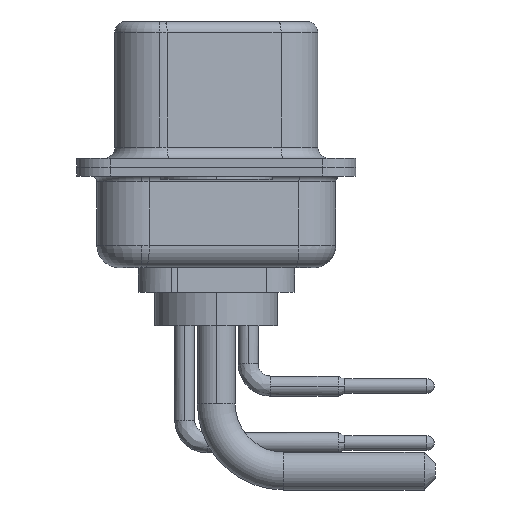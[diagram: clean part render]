
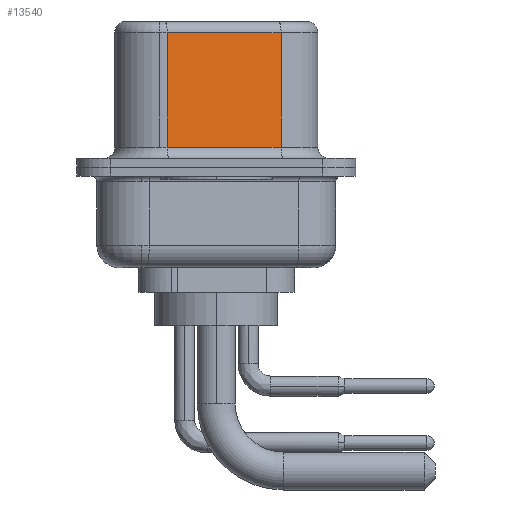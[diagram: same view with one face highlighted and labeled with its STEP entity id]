
A CAD part, left-side view. The second image highlights one B-rep face of the part: STEP entity #13540.
In plain terms, the highlighted planar face has unit normal (-0.985, -0.174, 0).
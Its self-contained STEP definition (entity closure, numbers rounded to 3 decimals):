
#1412 = EDGE_CURVE ( 'NONE', #9887, #16896, #6601, .T. ) ;
#1560 = DIRECTION ( 'NONE',  ( 0., 0., -1. ) ) ;
#3458 = PLANE ( 'NONE',  #9472 ) ;
#3875 = DIRECTION ( 'NONE',  ( -0.174, 0.985, 0. ) ) ;
#4397 = DIRECTION ( 'NONE',  ( 0.174, -0.985, 0. ) ) ;
#4495 = CARTESIAN_POINT ( 'NONE',  ( 3.68, 2.203, 6.02 ) ) ;
#4924 = CARTESIAN_POINT ( 'NONE',  ( 4.58, -2.897, 6.52 ) ) ;
#5695 = ORIENTED_EDGE ( 'NONE', *, *, #16134, .T. ) ;
#6601 = LINE ( 'NONE', #11292, #7530 ) ;
#6937 = ORIENTED_EDGE ( 'NONE', *, *, #1412, .T. ) ;
#7530 = VECTOR ( 'NONE', #15975, 1000. ) ;
#7934 = CARTESIAN_POINT ( 'NONE',  ( 4.58, -2.897, 6.02 ) ) ;
#8263 = DIRECTION ( 'NONE',  ( 0.985, 0.174, 0. ) ) ;
#9199 = ORIENTED_EDGE ( 'NONE', *, *, #12507, .T. ) ;
#9436 = VECTOR ( 'NONE', #4397, 1000. ) ;
#9472 = AXIS2_PLACEMENT_3D ( 'NONE', #16198, #8263, #3875 ) ;
#9713 = LINE ( 'NONE', #4924, #14267 ) ;
#9887 = VERTEX_POINT ( 'NONE', #7934 ) ;
#10927 = VERTEX_POINT ( 'NONE', #16264 ) ;
#11241 = ORIENTED_EDGE ( 'NONE', *, *, #18923, .F. ) ;
#11292 = CARTESIAN_POINT ( 'NONE',  ( 4.58, -2.897, 6.02 ) ) ;
#12507 = EDGE_CURVE ( 'NONE', #17890, #10927, #18565, .T. ) ;
#12508 = VECTOR ( 'NONE', #14030, 1000. ) ;
#12582 = CARTESIAN_POINT ( 'NONE',  ( 3.68, 2.203, 6.52 ) ) ;
#13540 = ADVANCED_FACE ( 'NONE', ( #17644 ), #3458, .F. ) ;
#14030 = DIRECTION ( 'NONE',  ( 0., 0., -1. ) ) ;
#14267 = VECTOR ( 'NONE', #1560, 1000. ) ;
#15975 = DIRECTION ( 'NONE',  ( -0.174, 0.985, 0. ) ) ;
#16134 = EDGE_CURVE ( 'NONE', #16896, #17890, #20601, .T. ) ;
#16198 = CARTESIAN_POINT ( 'NONE',  ( 4.58, -2.897, 6.52 ) ) ;
#16264 = CARTESIAN_POINT ( 'NONE',  ( 4.58, -2.897, 0.9 ) ) ;
#16656 = EDGE_LOOP ( 'NONE', ( #11241, #6937, #5695, #9199 ) ) ;
#16690 = CARTESIAN_POINT ( 'NONE',  ( 3.68, 2.203, 0.9 ) ) ;
#16896 = VERTEX_POINT ( 'NONE', #4495 ) ;
#17305 = CARTESIAN_POINT ( 'NONE',  ( 4.58, -2.897, 0.9 ) ) ;
#17644 = FACE_OUTER_BOUND ( 'NONE', #16656, .T. ) ;
#17890 = VERTEX_POINT ( 'NONE', #16690 ) ;
#18565 = LINE ( 'NONE', #17305, #9436 ) ;
#18923 = EDGE_CURVE ( 'NONE', #9887, #10927, #9713, .T. ) ;
#20601 = LINE ( 'NONE', #12582, #12508 ) ;
